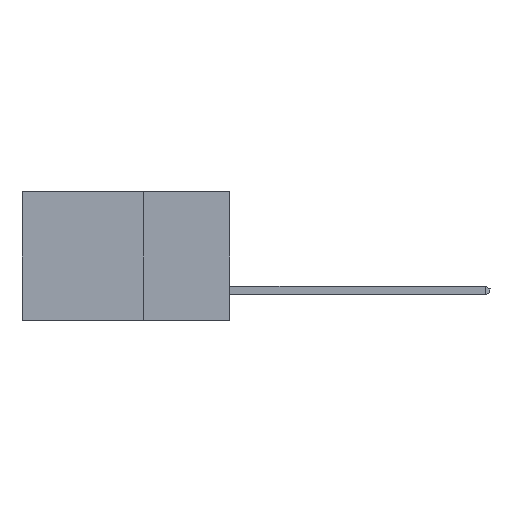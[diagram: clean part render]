
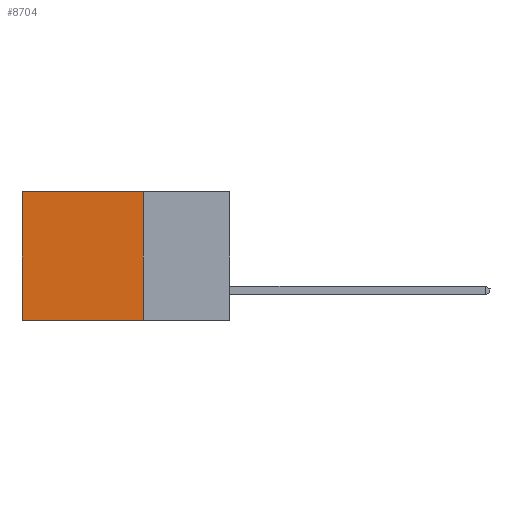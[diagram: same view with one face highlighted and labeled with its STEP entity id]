
A CAD part, left-side view. The second image highlights one B-rep face of the part: STEP entity #8704.
In plain terms, the highlighted planar face has unit normal (-1, 0, 0).
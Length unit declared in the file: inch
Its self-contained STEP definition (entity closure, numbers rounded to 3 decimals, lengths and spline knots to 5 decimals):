
#155 = LINE ( 'NONE', #1238, #14177 ) ;
#281 = DIRECTION ( 'NONE',  ( 1., 0., 0. ) ) ;
#942 = CARTESIAN_POINT ( 'NONE',  ( 0.2615, 0.25, -0.37 ) ) ;
#1036 = VECTOR ( 'NONE', #15197, 39.37008 ) ;
#1095 = DIRECTION ( 'NONE',  ( 0., 0., -1. ) ) ;
#1152 = DIRECTION ( 'NONE',  ( 0., 0., -1. ) ) ;
#1238 = CARTESIAN_POINT ( 'NONE',  ( 0.2615, 0.25, -0.37 ) ) ;
#2264 = LINE ( 'NONE', #6933, #1036 ) ;
#2612 = EDGE_CURVE ( 'NONE', #8034, #5838, #155, .T. ) ;
#2914 = EDGE_CURVE ( 'NONE', #14559, #3177, #11822, .T. ) ;
#2988 = AXIS2_PLACEMENT_3D ( 'NONE', #7529, #281, #12283 ) ;
#3177 = VERTEX_POINT ( 'NONE', #6497 ) ;
#3704 = CARTESIAN_POINT ( 'NONE',  ( 0.2615, 0.25, 0. ) ) ;
#5414 = EDGE_LOOP ( 'NONE', ( #14375, #14253, #10972, #13947 ) ) ;
#5838 = VERTEX_POINT ( 'NONE', #6211 ) ;
#6211 = CARTESIAN_POINT ( 'NONE',  ( 0.2615, 0.25, -0.37 ) ) ;
#6497 = CARTESIAN_POINT ( 'NONE',  ( 0.2615, 0.6, -0.37 ) ) ;
#6933 = CARTESIAN_POINT ( 'NONE',  ( 0.2615, 0.25, 0. ) ) ;
#7335 = VECTOR ( 'NONE', #1152, 39.37008 ) ;
#7374 = EDGE_CURVE ( 'NONE', #8034, #14559, #2264, .T. ) ;
#7529 = CARTESIAN_POINT ( 'NONE',  ( 0.2615, 0.25, -0.37 ) ) ;
#8034 = VERTEX_POINT ( 'NONE', #3704 ) ;
#8230 = CARTESIAN_POINT ( 'NONE',  ( 0.2615, 0.6, -0.37 ) ) ;
#8704 = ADVANCED_FACE ( 'NONE', ( #14605 ), #12194, .F. ) ;
#10972 = ORIENTED_EDGE ( 'NONE', *, *, #2612, .F. ) ;
#11822 = LINE ( 'NONE', #8230, #7335 ) ;
#11853 = DIRECTION ( 'NONE',  ( 0., 1., 0. ) ) ;
#12102 = CARTESIAN_POINT ( 'NONE',  ( 0.2615, 0.6, 0. ) ) ;
#12194 = PLANE ( 'NONE',  #2988 ) ;
#12283 = DIRECTION ( 'NONE',  ( 0., 0., -1. ) ) ;
#13472 = EDGE_CURVE ( 'NONE', #5838, #3177, #15111, .T. ) ;
#13758 = VECTOR ( 'NONE', #11853, 39.37008 ) ;
#13947 = ORIENTED_EDGE ( 'NONE', *, *, #7374, .T. ) ;
#14177 = VECTOR ( 'NONE', #1095, 39.37008 ) ;
#14253 = ORIENTED_EDGE ( 'NONE', *, *, #13472, .F. ) ;
#14375 = ORIENTED_EDGE ( 'NONE', *, *, #2914, .T. ) ;
#14559 = VERTEX_POINT ( 'NONE', #12102 ) ;
#14605 = FACE_OUTER_BOUND ( 'NONE', #5414, .T. ) ;
#15111 = LINE ( 'NONE', #942, #13758 ) ;
#15197 = DIRECTION ( 'NONE',  ( 0., 1., 0. ) ) ;
